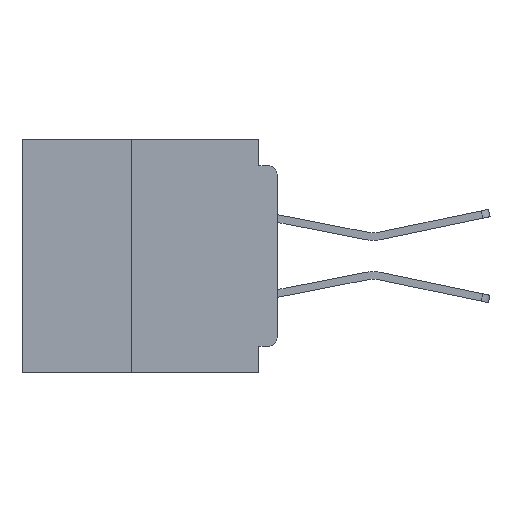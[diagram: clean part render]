
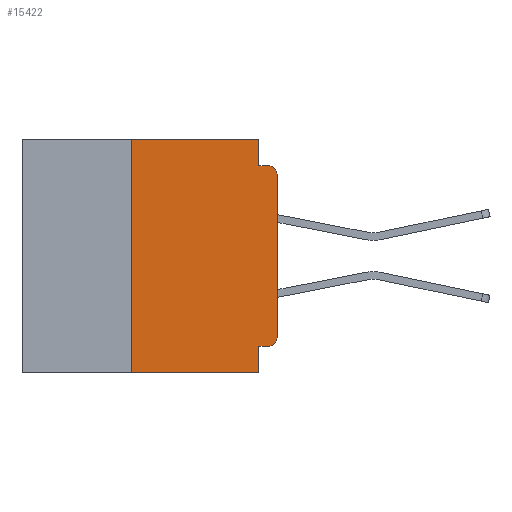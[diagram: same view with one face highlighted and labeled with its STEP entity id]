
A CAD part, left-side view. The second image highlights one B-rep face of the part: STEP entity #15422.
In plain terms, the highlighted planar face has unit normal (-1, 0, 0).
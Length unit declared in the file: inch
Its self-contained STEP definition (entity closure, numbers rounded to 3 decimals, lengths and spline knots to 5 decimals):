
#1242 = EDGE_CURVE ( 'NONE', #40687, #38855, #45297, .T. ) ;
#2036 = CARTESIAN_POINT ( 'NONE',  ( 0., 0.015, -0.34 ) ) ;
#2944 = VERTEX_POINT ( 'NONE', #23709 ) ;
#3082 = VECTOR ( 'NONE', #35055, 39.37008 ) ;
#3369 = VECTOR ( 'NONE', #4789, 39.37008 ) ;
#3417 = EDGE_CURVE ( 'NONE', #22405, #44484, #35225, .T. ) ;
#3475 = LINE ( 'NONE', #32748, #11959 ) ;
#3486 = AXIS2_PLACEMENT_3D ( 'NONE', #2036, #31416, #6284 ) ;
#3990 = VERTEX_POINT ( 'NONE', #51799 ) ;
#4010 = CARTESIAN_POINT ( 'NONE',  ( 0., 0.031, -0.355 ) ) ;
#4360 = ORIENTED_EDGE ( 'NONE', *, *, #34336, .F. ) ;
#4713 = CIRCLE ( 'NONE', #3486, 0.015 ) ;
#4789 = DIRECTION ( 'NONE',  ( 0., -1., 0. ) ) ;
#5156 = CARTESIAN_POINT ( 'NONE',  ( 0., 0.437, 0. ) ) ;
#5198 = EDGE_CURVE ( 'NONE', #2944, #3990, #27235, .T. ) ;
#5630 = CARTESIAN_POINT ( 'NONE',  ( 0., 0.015, -0.355 ) ) ;
#5747 = CARTESIAN_POINT ( 'NONE',  ( 0., 0., -0.355 ) ) ;
#5761 = LINE ( 'NONE', #42292, #37897 ) ;
#6284 = DIRECTION ( 'NONE',  ( 0., 0., -1. ) ) ;
#6789 = DIRECTION ( 'NONE',  ( 0., -1., 0. ) ) ;
#9009 = CARTESIAN_POINT ( 'NONE',  ( 0., 0.437, -0.4 ) ) ;
#9352 = DIRECTION ( 'NONE',  ( 1., 0., 0. ) ) ;
#11959 = VECTOR ( 'NONE', #20444, 39.37008 ) ;
#12606 = DIRECTION ( 'NONE',  ( -1., 0., 0. ) ) ;
#13901 = AXIS2_PLACEMENT_3D ( 'NONE', #37761, #12606, #41987 ) ;
#14339 = LINE ( 'NONE', #52528, #36671 ) ;
#15422 = ADVANCED_FACE ( 'NONE', ( #45878 ), #42730, .F. ) ;
#15795 = DIRECTION ( 'NONE',  ( 0., 0., 1. ) ) ;
#16769 = VERTEX_POINT ( 'NONE', #52474 ) ;
#19831 = DIRECTION ( 'NONE',  ( 0., 0., -1. ) ) ;
#20253 = CARTESIAN_POINT ( 'NONE',  ( 0., 0.031, 0. ) ) ;
#20444 = DIRECTION ( 'NONE',  ( 0., -1., 0. ) ) ;
#20656 = CARTESIAN_POINT ( 'NONE',  ( 0., 0.031, 0. ) ) ;
#20772 = ORIENTED_EDGE ( 'NONE', *, *, #5198, .T. ) ;
#22405 = VERTEX_POINT ( 'NONE', #5630 ) ;
#22985 = VECTOR ( 'NONE', #19831, 39.37008 ) ;
#23709 = CARTESIAN_POINT ( 'NONE',  ( 0., 0., -0.34 ) ) ;
#24131 = ORIENTED_EDGE ( 'NONE', *, *, #46593, .T. ) ;
#24963 = VERTEX_POINT ( 'NONE', #32899 ) ;
#25589 = DIRECTION ( 'NONE',  ( 0., 0., -1. ) ) ;
#25846 = VERTEX_POINT ( 'NONE', #30105 ) ;
#26990 = LINE ( 'NONE', #9009, #3369 ) ;
#27235 = LINE ( 'NONE', #35211, #48175 ) ;
#28895 = VERTEX_POINT ( 'NONE', #54101 ) ;
#29648 = ORIENTED_EDGE ( 'NONE', *, *, #29783, .T. ) ;
#29783 = EDGE_CURVE ( 'NONE', #22405, #2944, #4713, .T. ) ;
#30105 = CARTESIAN_POINT ( 'NONE',  ( 0., 0.015, -0.045 ) ) ;
#31416 = DIRECTION ( 'NONE',  ( -1., 0., 0. ) ) ;
#31479 = VECTOR ( 'NONE', #15795, 39.37008 ) ;
#32748 = CARTESIAN_POINT ( 'NONE',  ( 0., 0.437, 0. ) ) ;
#32899 = CARTESIAN_POINT ( 'NONE',  ( 0., 0.25, -0.4 ) ) ;
#33973 = EDGE_CURVE ( 'NONE', #24963, #16769, #43922, .T. ) ;
#34336 = EDGE_CURVE ( 'NONE', #38855, #25846, #14339, .T. ) ;
#35055 = DIRECTION ( 'NONE',  ( 0., 1., 0. ) ) ;
#35151 = EDGE_CURVE ( 'NONE', #44484, #28895, #5761, .T. ) ;
#35211 = CARTESIAN_POINT ( 'NONE',  ( 0., 0., 0. ) ) ;
#35225 = LINE ( 'NONE', #5747, #3082 ) ;
#35380 = ORIENTED_EDGE ( 'NONE', *, *, #3417, .F. ) ;
#36428 = CIRCLE ( 'NONE', #13901, 0.015 ) ;
#36671 = VECTOR ( 'NONE', #6789, 39.37008 ) ;
#37058 = ORIENTED_EDGE ( 'NONE', *, *, #35151, .F. ) ;
#37421 = ORIENTED_EDGE ( 'NONE', *, *, #1242, .F. ) ;
#37603 = ORIENTED_EDGE ( 'NONE', *, *, #49724, .T. ) ;
#37761 = CARTESIAN_POINT ( 'NONE',  ( 0., 0.015, -0.06 ) ) ;
#37897 = VECTOR ( 'NONE', #25589, 39.37008 ) ;
#38701 = DIRECTION ( 'NONE',  ( 0., 0., -1. ) ) ;
#38855 = VERTEX_POINT ( 'NONE', #45953 ) ;
#40687 = VERTEX_POINT ( 'NONE', #20253 ) ;
#41987 = DIRECTION ( 'NONE',  ( 0., 0., -1. ) ) ;
#42292 = CARTESIAN_POINT ( 'NONE',  ( 0., 0.031, -0.4 ) ) ;
#42730 = PLANE ( 'NONE',  #53541 ) ;
#43922 = LINE ( 'NONE', #46208, #31479 ) ;
#44484 = VERTEX_POINT ( 'NONE', #4010 ) ;
#45297 = LINE ( 'NONE', #20656, #22985 ) ;
#45878 = FACE_OUTER_BOUND ( 'NONE', #51820, .T. ) ;
#45953 = CARTESIAN_POINT ( 'NONE',  ( 0., 0.031, -0.045 ) ) ;
#46208 = CARTESIAN_POINT ( 'NONE',  ( 0., 0.25, -0.4 ) ) ;
#46593 = EDGE_CURVE ( 'NONE', #3990, #25846, #36428, .T. ) ;
#47811 = DIRECTION ( 'NONE',  ( 0., 0., 1. ) ) ;
#48175 = VECTOR ( 'NONE', #47811, 39.37008 ) ;
#48735 = ORIENTED_EDGE ( 'NONE', *, *, #33973, .F. ) ;
#48835 = EDGE_CURVE ( 'NONE', #16769, #40687, #3475, .T. ) ;
#49724 = EDGE_CURVE ( 'NONE', #24963, #28895, #26990, .T. ) ;
#50217 = ORIENTED_EDGE ( 'NONE', *, *, #48835, .F. ) ;
#51799 = CARTESIAN_POINT ( 'NONE',  ( 0., 0., -0.06 ) ) ;
#51820 = EDGE_LOOP ( 'NONE', ( #20772, #24131, #4360, #37421, #50217, #48735, #37603, #37058, #35380, #29648 ) ) ;
#52474 = CARTESIAN_POINT ( 'NONE',  ( 0., 0.25, 0. ) ) ;
#52528 = CARTESIAN_POINT ( 'NONE',  ( 0., 0., -0.045 ) ) ;
#53541 = AXIS2_PLACEMENT_3D ( 'NONE', #5156, #9352, #38701 ) ;
#54101 = CARTESIAN_POINT ( 'NONE',  ( 0., 0.031, -0.4 ) ) ;
